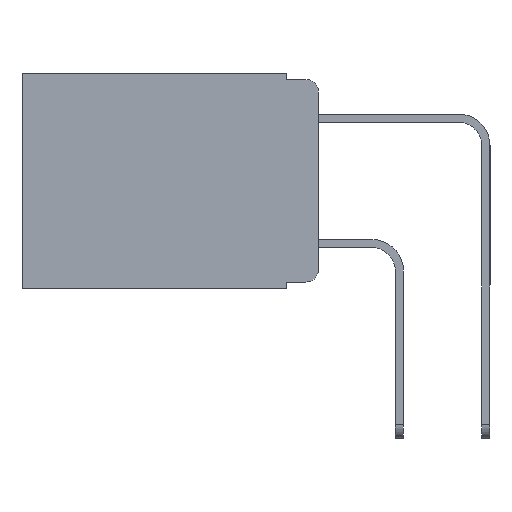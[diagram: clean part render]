
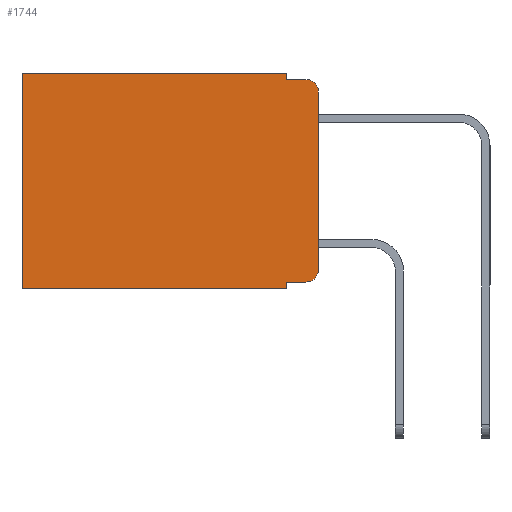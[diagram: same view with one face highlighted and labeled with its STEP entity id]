
A CAD part, left-side view. The second image highlights one B-rep face of the part: STEP entity #1744.
In plain terms, the highlighted planar face has unit normal (-1, 0, 0).
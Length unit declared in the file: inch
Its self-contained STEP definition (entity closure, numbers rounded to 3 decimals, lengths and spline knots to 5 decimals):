
#60 = DIRECTION ( 'NONE',  ( 0., 1., 0. ) ) ;
#227 = AXIS2_PLACEMENT_3D ( 'NONE', #11364, #9519, #10834 ) ;
#853 = LINE ( 'NONE', #3504, #15040 ) ;
#889 = EDGE_CURVE ( 'NONE', #3238, #8630, #2345, .T. ) ;
#1437 = DIRECTION ( 'NONE',  ( 0., 0., -1. ) ) ;
#1536 = CARTESIAN_POINT ( 'NONE',  ( 0.298, 0.02, -0.333 ) ) ;
#1744 = ADVANCED_FACE ( 'NONE', ( #18163 ), #3449, .F. ) ;
#1954 = VERTEX_POINT ( 'NONE', #14197 ) ;
#1982 = ORIENTED_EDGE ( 'NONE', *, *, #16342, .F. ) ;
#2111 = CARTESIAN_POINT ( 'NONE',  ( 0.298, 0.051, 0. ) ) ;
#2214 = CARTESIAN_POINT ( 'NONE',  ( 0.298, 0.051, -0.333 ) ) ;
#2342 = LINE ( 'NONE', #4704, #13120 ) ;
#2345 = CIRCLE ( 'NONE', #227, 0.02 ) ;
#2647 = VECTOR ( 'NONE', #1437, 39.37008 ) ;
#3019 = CIRCLE ( 'NONE', #14369, 0.02 ) ;
#3238 = VERTEX_POINT ( 'NONE', #15092 ) ;
#3449 = PLANE ( 'NONE',  #5929 ) ;
#3504 = CARTESIAN_POINT ( 'NONE',  ( 0.298, 0.051, 0. ) ) ;
#3602 = ORIENTED_EDGE ( 'NONE', *, *, #16152, .T. ) ;
#3909 = EDGE_CURVE ( 'NONE', #3238, #1954, #13494, .T. ) ;
#3966 = CARTESIAN_POINT ( 'NONE',  ( 0.298, 0., 0. ) ) ;
#4051 = ORIENTED_EDGE ( 'NONE', *, *, #15453, .T. ) ;
#4159 = CARTESIAN_POINT ( 'NONE',  ( 0.298, 0.473, 0. ) ) ;
#4704 = CARTESIAN_POINT ( 'NONE',  ( 0.298, 0.473, 0. ) ) ;
#4845 = VERTEX_POINT ( 'NONE', #2214 ) ;
#4975 = CARTESIAN_POINT ( 'NONE',  ( 0.298, 0.473, -0.343 ) ) ;
#5929 = AXIS2_PLACEMENT_3D ( 'NONE', #3966, #8730, #9418 ) ;
#6000 = LINE ( 'NONE', #7087, #9634 ) ;
#6080 = DIRECTION ( 'NONE',  ( -1., 0., 0. ) ) ;
#6082 = DIRECTION ( 'NONE',  ( 0., 0., -1. ) ) ;
#6501 = VECTOR ( 'NONE', #60, 39.37008 ) ;
#6647 = ORIENTED_EDGE ( 'NONE', *, *, #15030, .F. ) ;
#6924 = LINE ( 'NONE', #7319, #6501 ) ;
#7087 = CARTESIAN_POINT ( 'NONE',  ( 0.298, 0.051, -0.01 ) ) ;
#7099 = VECTOR ( 'NONE', #10460, 39.37008 ) ;
#7238 = LINE ( 'NONE', #9853, #2647 ) ;
#7319 = CARTESIAN_POINT ( 'NONE',  ( 0.298, 0., 0. ) ) ;
#7533 = LINE ( 'NONE', #9145, #7099 ) ;
#8000 = CARTESIAN_POINT ( 'NONE',  ( 0.298, 0., -0.343 ) ) ;
#8134 = ORIENTED_EDGE ( 'NONE', *, *, #889, .T. ) ;
#8630 = VERTEX_POINT ( 'NONE', #12059 ) ;
#8730 = DIRECTION ( 'NONE',  ( 1., 0., 0. ) ) ;
#9145 = CARTESIAN_POINT ( 'NONE',  ( 0.298, 0.051, -0.333 ) ) ;
#9245 = CARTESIAN_POINT ( 'NONE',  ( 0.298, 0., 0. ) ) ;
#9335 = VERTEX_POINT ( 'NONE', #2111 ) ;
#9366 = DIRECTION ( 'NONE',  ( 0., 1., 0. ) ) ;
#9418 = DIRECTION ( 'NONE',  ( 0., 0., -1. ) ) ;
#9519 = DIRECTION ( 'NONE',  ( -1., 0., 0. ) ) ;
#9634 = VECTOR ( 'NONE', #18139, 39.37008 ) ;
#9652 = VECTOR ( 'NONE', #12104, 39.37008 ) ;
#9853 = CARTESIAN_POINT ( 'NONE',  ( 0.298, 0.051, 0. ) ) ;
#10409 = LINE ( 'NONE', #8000, #16997 ) ;
#10460 = DIRECTION ( 'NONE',  ( 0., -1., 0. ) ) ;
#10700 = ORIENTED_EDGE ( 'NONE', *, *, #12663, .T. ) ;
#10834 = DIRECTION ( 'NONE',  ( 0., 0., -1. ) ) ;
#11364 = CARTESIAN_POINT ( 'NONE',  ( 0.298, 0.02, -0.03 ) ) ;
#11652 = EDGE_CURVE ( 'NONE', #16150, #1954, #3019, .T. ) ;
#12020 = EDGE_LOOP ( 'NONE', ( #16015, #8134, #13701, #1982, #3602, #4051, #6647, #17881, #10700, #14980 ) ) ;
#12059 = CARTESIAN_POINT ( 'NONE',  ( 0.298, 0.02, -0.01 ) ) ;
#12104 = DIRECTION ( 'NONE',  ( 0., 0., -1. ) ) ;
#12663 = EDGE_CURVE ( 'NONE', #4845, #16150, #7533, .T. ) ;
#12757 = VERTEX_POINT ( 'NONE', #17775 ) ;
#13120 = VECTOR ( 'NONE', #6082, 39.37008 ) ;
#13303 = DIRECTION ( 'NONE',  ( 0., 0., -1. ) ) ;
#13494 = LINE ( 'NONE', #9245, #9652 ) ;
#13701 = ORIENTED_EDGE ( 'NONE', *, *, #18132, .F. ) ;
#14197 = CARTESIAN_POINT ( 'NONE',  ( 0.298, 0., -0.313 ) ) ;
#14369 = AXIS2_PLACEMENT_3D ( 'NONE', #14477, #6080, #15822 ) ;
#14477 = CARTESIAN_POINT ( 'NONE',  ( 0.298, 0.02, -0.313 ) ) ;
#14563 = EDGE_CURVE ( 'NONE', #4845, #16363, #7238, .T. ) ;
#14980 = ORIENTED_EDGE ( 'NONE', *, *, #11652, .T. ) ;
#15030 = EDGE_CURVE ( 'NONE', #16363, #16387, #10409, .T. ) ;
#15040 = VECTOR ( 'NONE', #13303, 39.37008 ) ;
#15092 = CARTESIAN_POINT ( 'NONE',  ( 0.298, 0., -0.03 ) ) ;
#15453 = EDGE_CURVE ( 'NONE', #17404, #16387, #2342, .T. ) ;
#15822 = DIRECTION ( 'NONE',  ( 0., 0., -1. ) ) ;
#16015 = ORIENTED_EDGE ( 'NONE', *, *, #3909, .F. ) ;
#16035 = CARTESIAN_POINT ( 'NONE',  ( 0.298, 0.051, -0.343 ) ) ;
#16150 = VERTEX_POINT ( 'NONE', #1536 ) ;
#16152 = EDGE_CURVE ( 'NONE', #9335, #17404, #6924, .T. ) ;
#16342 = EDGE_CURVE ( 'NONE', #9335, #12757, #853, .T. ) ;
#16363 = VERTEX_POINT ( 'NONE', #16035 ) ;
#16387 = VERTEX_POINT ( 'NONE', #4975 ) ;
#16997 = VECTOR ( 'NONE', #9366, 39.37008 ) ;
#17404 = VERTEX_POINT ( 'NONE', #4159 ) ;
#17775 = CARTESIAN_POINT ( 'NONE',  ( 0.298, 0.051, -0.01 ) ) ;
#17881 = ORIENTED_EDGE ( 'NONE', *, *, #14563, .F. ) ;
#18132 = EDGE_CURVE ( 'NONE', #12757, #8630, #6000, .T. ) ;
#18139 = DIRECTION ( 'NONE',  ( 0., -1., 0. ) ) ;
#18163 = FACE_OUTER_BOUND ( 'NONE', #12020, .T. ) ;
